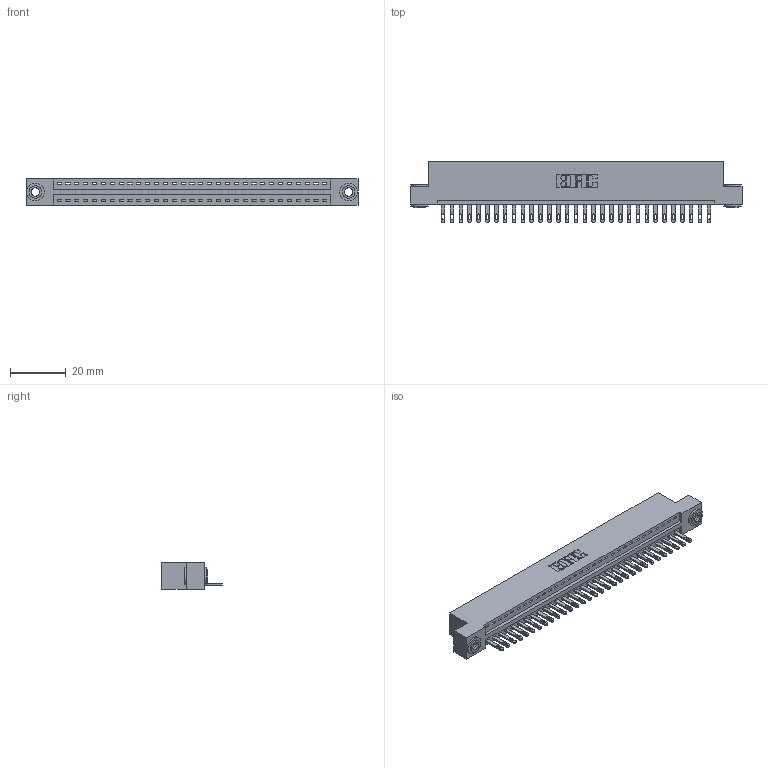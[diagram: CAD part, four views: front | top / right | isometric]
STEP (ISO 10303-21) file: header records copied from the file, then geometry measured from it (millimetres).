
FILE_DESCRIPTION (( 'STEP AP203' ), '1' );
FILE_NAME ('346-031-500-103.STEP', '2022-05-06T16:21:21', ( '' ), ( '' ), 'SwSTEP 2.0', 'SolidWorks 2020', '' );
FILE_SCHEMA (( 'CONFIG_CONTROL_DESIGN' ));
Length unit declared in the file: inch
Products named in the file (4): 345-250-002_345-250-002-102; 345-292-001_345-293-100; 346 Part_Flush Mounting Lugs - 0.156 Dia-TH; 346-031-500-103
Assembly tree (34 placements, depth 2):
  346-031-500-103
    346 Part_Flush Mounting Lugs - 0.156 Dia-TH
    345-292-001_345-293-100  x31
    345-250-002_345-250-002-102  x2
Bounding box: 119 x 21.84 x 9.4 mm (x, y, z)
Volume: 11335.5 mm3; surface area: 14373 mm2
Topology: 34 solids, 34 shells, 1848 faces, 5649 edges, 3762 vertices
Faces by surface type: plane 1154, cylinder 686, cone 8
Entity records: 21716 total; most frequent: CARTESIAN_POINT 3706, ORIENTED_EDGE 3662, DIRECTION 3315, EDGE_CURVE 1831, VECTOR 1547, LINE 1547, VERTEX_POINT 1218, AXIS2_PLACEMENT_3D 884
